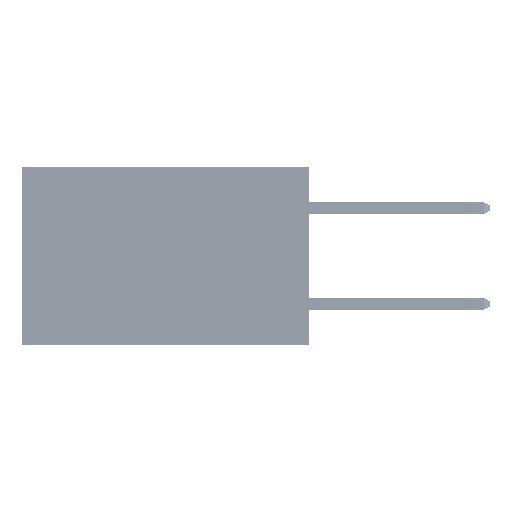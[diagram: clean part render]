
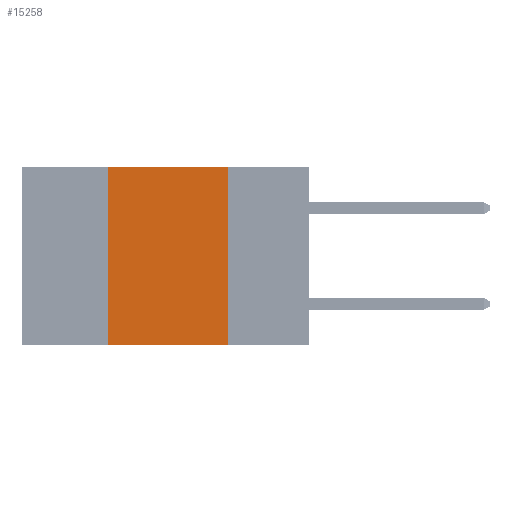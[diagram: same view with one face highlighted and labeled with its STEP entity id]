
A CAD part, left-side view. The second image highlights one B-rep face of the part: STEP entity #15258.
In plain terms, the highlighted planar face has unit normal (-1, 0, 0).
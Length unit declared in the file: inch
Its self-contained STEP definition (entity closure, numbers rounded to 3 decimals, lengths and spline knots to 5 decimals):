
#1182 = VERTEX_POINT ( 'NONE', #36709 ) ;
#1255 = ORIENTED_EDGE ( 'NONE', *, *, #36239, .F. ) ;
#4402 = AXIS2_PLACEMENT_3D ( 'NONE', #31410, #23393, #35150 ) ;
#6369 = ORIENTED_EDGE ( 'NONE', *, *, #36149, .T. ) ;
#8824 = FACE_OUTER_BOUND ( 'NONE', #21503, .T. ) ;
#9845 = LINE ( 'NONE', #25927, #10411 ) ;
#9916 = VERTEX_POINT ( 'NONE', #34903 ) ;
#10411 = VECTOR ( 'NONE', #14654, 39.37008 ) ;
#10581 = VERTEX_POINT ( 'NONE', #37661 ) ;
#10882 = VERTEX_POINT ( 'NONE', #21465 ) ;
#14001 = LINE ( 'NONE', #41690, #38016 ) ;
#14654 = DIRECTION ( 'NONE',  ( 0., -1., 0. ) ) ;
#15258 = ADVANCED_FACE ( 'NONE', ( #8824 ), #45863, .F. ) ;
#17438 = CARTESIAN_POINT ( 'NONE',  ( 0., 0.6, -0.37 ) ) ;
#19392 = DIRECTION ( 'NONE',  ( 0., 0., -1. ) ) ;
#19808 = LINE ( 'NONE', #17438, #31525 ) ;
#19925 = DIRECTION ( 'NONE',  ( 0., 0., 1. ) ) ;
#21465 = CARTESIAN_POINT ( 'NONE',  ( 0., 0.17, 0. ) ) ;
#21503 = EDGE_LOOP ( 'NONE', ( #42280, #1255, #27742, #6369 ) ) ;
#22284 = EDGE_CURVE ( 'NONE', #10581, #9916, #33313, .T. ) ;
#23062 = CARTESIAN_POINT ( 'NONE',  ( 0., 0.42, 0. ) ) ;
#23393 = DIRECTION ( 'NONE',  ( 1., 0., 0. ) ) ;
#25927 = CARTESIAN_POINT ( 'NONE',  ( 0., 0.6, 0. ) ) ;
#27742 = ORIENTED_EDGE ( 'NONE', *, *, #22284, .F. ) ;
#31410 = CARTESIAN_POINT ( 'NONE',  ( 0., 0.6, 0. ) ) ;
#31525 = VECTOR ( 'NONE', #39880, 39.37008 ) ;
#33313 = LINE ( 'NONE', #23062, #33865 ) ;
#33865 = VECTOR ( 'NONE', #19925, 39.37008 ) ;
#34903 = CARTESIAN_POINT ( 'NONE',  ( 0., 0.42, 0. ) ) ;
#35150 = DIRECTION ( 'NONE',  ( 0., 0., -1. ) ) ;
#36149 = EDGE_CURVE ( 'NONE', #10581, #1182, #19808, .T. ) ;
#36239 = EDGE_CURVE ( 'NONE', #9916, #10882, #9845, .T. ) ;
#36709 = CARTESIAN_POINT ( 'NONE',  ( 0., 0.17, -0.37 ) ) ;
#37661 = CARTESIAN_POINT ( 'NONE',  ( 0., 0.42, -0.37 ) ) ;
#38016 = VECTOR ( 'NONE', #19392, 39.37008 ) ;
#39880 = DIRECTION ( 'NONE',  ( 0., -1., 0. ) ) ;
#40835 = EDGE_CURVE ( 'NONE', #10882, #1182, #14001, .T. ) ;
#41690 = CARTESIAN_POINT ( 'NONE',  ( 0., 0.17, 0. ) ) ;
#42280 = ORIENTED_EDGE ( 'NONE', *, *, #40835, .F. ) ;
#45863 = PLANE ( 'NONE',  #4402 ) ;
